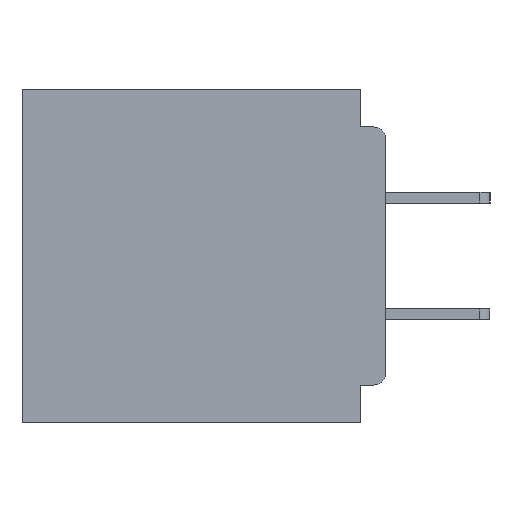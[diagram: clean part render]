
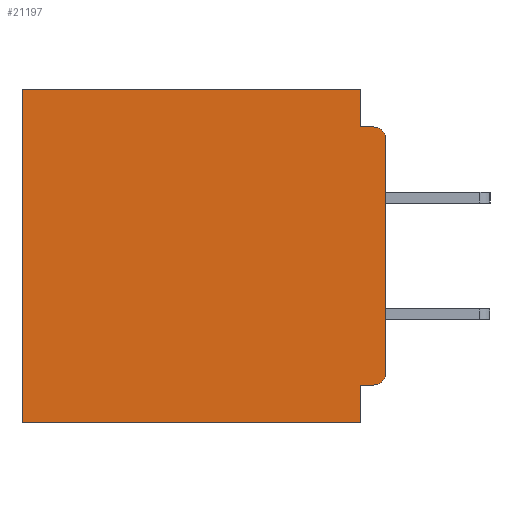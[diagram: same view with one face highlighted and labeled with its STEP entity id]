
A CAD part, left-side view. The second image highlights one B-rep face of the part: STEP entity #21197.
In plain terms, the highlighted planar face has unit normal (-1, 0, 0).
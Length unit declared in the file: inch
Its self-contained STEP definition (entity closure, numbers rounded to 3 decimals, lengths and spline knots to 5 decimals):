
#126 = CARTESIAN_POINT ( 'NONE',  ( 0.3, 0.015, -0.355 ) ) ;
#227 = ORIENTED_EDGE ( 'NONE', *, *, #52758, .F. ) ;
#701 = VERTEX_POINT ( 'NONE', #29781 ) ;
#1132 = CARTESIAN_POINT ( 'NONE',  ( 0.3, 0., -0.355 ) ) ;
#1779 = DIRECTION ( 'NONE',  ( 0., 0., -1. ) ) ;
#2162 = LINE ( 'NONE', #1132, #40719 ) ;
#4245 = EDGE_CURVE ( 'NONE', #4622, #21391, #48327, .T. ) ;
#4622 = VERTEX_POINT ( 'NONE', #47290 ) ;
#5702 = DIRECTION ( 'NONE',  ( 1., 0., 0. ) ) ;
#5992 = DIRECTION ( 'NONE',  ( 0., 1., 0. ) ) ;
#6003 = VERTEX_POINT ( 'NONE', #43584 ) ;
#6024 = DIRECTION ( 'NONE',  ( 0., 1., 0. ) ) ;
#6478 = CARTESIAN_POINT ( 'NONE',  ( 0.3, 0.437, -0.4 ) ) ;
#6926 = VERTEX_POINT ( 'NONE', #43827 ) ;
#9029 = ORIENTED_EDGE ( 'NONE', *, *, #25541, .F. ) ;
#11813 = CARTESIAN_POINT ( 'NONE',  ( 0.3, 0.031, 0. ) ) ;
#11913 = ORIENTED_EDGE ( 'NONE', *, *, #37233, .T. ) ;
#11996 = CARTESIAN_POINT ( 'NONE',  ( 0.3, 0.015, -0.045 ) ) ;
#15191 = CARTESIAN_POINT ( 'NONE',  ( 0.3, 0., -0.4 ) ) ;
#15806 = CARTESIAN_POINT ( 'NONE',  ( 0.3, 0.031, 0. ) ) ;
#15816 = VERTEX_POINT ( 'NONE', #20514 ) ;
#16672 = AXIS2_PLACEMENT_3D ( 'NONE', #50210, #21335, #55010 ) ;
#19544 = CARTESIAN_POINT ( 'NONE',  ( 0.3, 0., 0. ) ) ;
#19690 = VECTOR ( 'NONE', #35860, 39.37008 ) ;
#19745 = DIRECTION ( 'NONE',  ( 0., 1., 0. ) ) ;
#19760 = VERTEX_POINT ( 'NONE', #126 ) ;
#19970 = EDGE_CURVE ( 'NONE', #6926, #21391, #60945, .T. ) ;
#20514 = CARTESIAN_POINT ( 'NONE',  ( 0.3, 0.031, -0.045 ) ) ;
#21026 = DIRECTION ( 'NONE',  ( 0., 0., -1. ) ) ;
#21105 = AXIS2_PLACEMENT_3D ( 'NONE', #15191, #5702, #39454 ) ;
#21197 = ADVANCED_FACE ( 'NONE', ( #44750 ), #34585, .F. ) ;
#21335 = DIRECTION ( 'NONE',  ( -1., 0., 0. ) ) ;
#21391 = VERTEX_POINT ( 'NONE', #53811 ) ;
#21492 = CARTESIAN_POINT ( 'NONE',  ( 0.3, 0., -0.4 ) ) ;
#21524 = DIRECTION ( 'NONE',  ( 0., 0., -1. ) ) ;
#21590 = EDGE_CURVE ( 'NONE', #19760, #701, #49188, .T. ) ;
#22187 = LINE ( 'NONE', #21492, #33470 ) ;
#22372 = VECTOR ( 'NONE', #21524, 39.37008 ) ;
#22656 = ORIENTED_EDGE ( 'NONE', *, *, #34588, .F. ) ;
#24875 = VERTEX_POINT ( 'NONE', #45859 ) ;
#25541 = EDGE_CURVE ( 'NONE', #57210, #15816, #59860, .T. ) ;
#25851 = CARTESIAN_POINT ( 'NONE',  ( 0.3, 0.031, -0.4 ) ) ;
#26556 = ORIENTED_EDGE ( 'NONE', *, *, #58680, .T. ) ;
#27656 = CARTESIAN_POINT ( 'NONE',  ( 0.3, 0.015, -0.06 ) ) ;
#28114 = AXIS2_PLACEMENT_3D ( 'NONE', #27656, #61273, #32519 ) ;
#29477 = EDGE_LOOP ( 'NONE', ( #227, #26556, #52173, #9029, #11913, #59213, #44001, #22656, #47545, #34811 ) ) ;
#29781 = CARTESIAN_POINT ( 'NONE',  ( 0.3, 0., -0.34 ) ) ;
#32519 = DIRECTION ( 'NONE',  ( 0., 0., -1. ) ) ;
#33470 = VECTOR ( 'NONE', #55170, 39.37008 ) ;
#33989 = VECTOR ( 'NONE', #5992, 39.37008 ) ;
#34491 = VECTOR ( 'NONE', #19745, 39.37008 ) ;
#34585 = PLANE ( 'NONE',  #21105 ) ;
#34588 = EDGE_CURVE ( 'NONE', #6003, #4622, #40260, .T. ) ;
#34811 = ORIENTED_EDGE ( 'NONE', *, *, #21590, .T. ) ;
#35860 = DIRECTION ( 'NONE',  ( 0., -1., 0. ) ) ;
#37233 = EDGE_CURVE ( 'NONE', #57210, #6926, #47336, .T. ) ;
#39454 = DIRECTION ( 'NONE',  ( 0., 0., -1. ) ) ;
#39752 = CARTESIAN_POINT ( 'NONE',  ( 0.3, 0., -0.4 ) ) ;
#40260 = LINE ( 'NONE', #25851, #51531 ) ;
#40719 = VECTOR ( 'NONE', #6024, 39.37008 ) ;
#43584 = CARTESIAN_POINT ( 'NONE',  ( 0.3, 0.031, -0.355 ) ) ;
#43827 = CARTESIAN_POINT ( 'NONE',  ( 0.3, 0.437, 0. ) ) ;
#44001 = ORIENTED_EDGE ( 'NONE', *, *, #4245, .F. ) ;
#44750 = FACE_OUTER_BOUND ( 'NONE', #29477, .T. ) ;
#45859 = CARTESIAN_POINT ( 'NONE',  ( 0.3, 0., -0.06 ) ) ;
#46852 = LINE ( 'NONE', #55406, #19690 ) ;
#47290 = CARTESIAN_POINT ( 'NONE',  ( 0.3, 0.031, -0.4 ) ) ;
#47336 = LINE ( 'NONE', #19544, #34491 ) ;
#47545 = ORIENTED_EDGE ( 'NONE', *, *, #50168, .F. ) ;
#48230 = VECTOR ( 'NONE', #21026, 39.37008 ) ;
#48327 = LINE ( 'NONE', #39752, #33989 ) ;
#49188 = CIRCLE ( 'NONE', #16672, 0.015 ) ;
#50168 = EDGE_CURVE ( 'NONE', #19760, #6003, #2162, .T. ) ;
#50210 = CARTESIAN_POINT ( 'NONE',  ( 0.3, 0.015, -0.34 ) ) ;
#51531 = VECTOR ( 'NONE', #1779, 39.37008 ) ;
#52173 = ORIENTED_EDGE ( 'NONE', *, *, #54281, .F. ) ;
#52758 = EDGE_CURVE ( 'NONE', #24875, #701, #22187, .T. ) ;
#53811 = CARTESIAN_POINT ( 'NONE',  ( 0.3, 0.437, -0.4 ) ) ;
#54281 = EDGE_CURVE ( 'NONE', #15816, #59608, #46852, .T. ) ;
#55010 = DIRECTION ( 'NONE',  ( 0., 0., -1. ) ) ;
#55170 = DIRECTION ( 'NONE',  ( 0., 0., -1. ) ) ;
#55406 = CARTESIAN_POINT ( 'NONE',  ( 0.3, 0., -0.045 ) ) ;
#57210 = VERTEX_POINT ( 'NONE', #15806 ) ;
#58680 = EDGE_CURVE ( 'NONE', #24875, #59608, #61718, .T. ) ;
#59213 = ORIENTED_EDGE ( 'NONE', *, *, #19970, .T. ) ;
#59608 = VERTEX_POINT ( 'NONE', #11996 ) ;
#59860 = LINE ( 'NONE', #11813, #22372 ) ;
#60945 = LINE ( 'NONE', #6478, #48230 ) ;
#61273 = DIRECTION ( 'NONE',  ( -1., 0., 0. ) ) ;
#61718 = CIRCLE ( 'NONE', #28114, 0.015 ) ;
